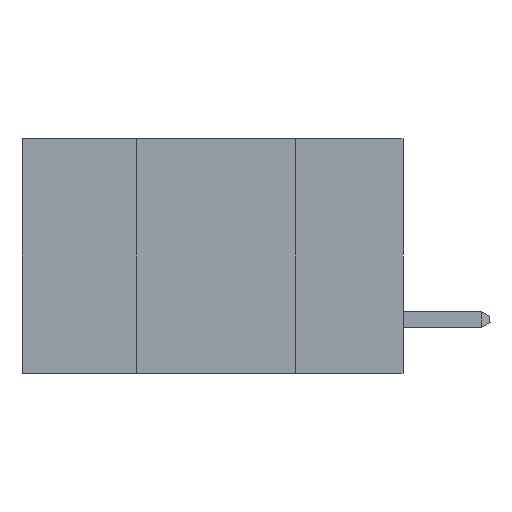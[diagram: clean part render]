
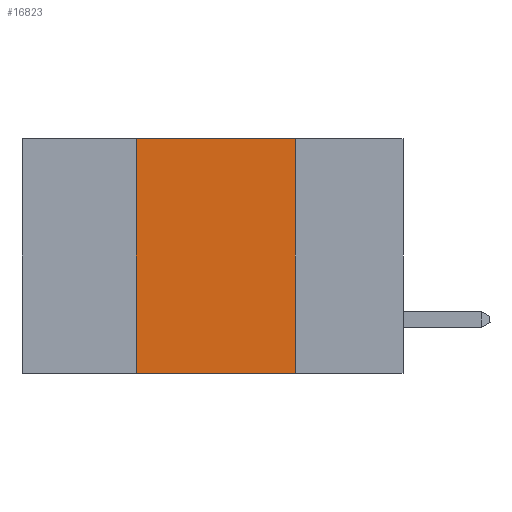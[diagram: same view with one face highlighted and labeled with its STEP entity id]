
A CAD part, left-side view. The second image highlights one B-rep face of the part: STEP entity #16823.
In plain terms, the highlighted planar face has unit normal (-1, 0, 0).
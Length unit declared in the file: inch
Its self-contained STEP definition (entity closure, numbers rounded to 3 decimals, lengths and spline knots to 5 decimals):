
#4189 = ORIENTED_EDGE ( 'NONE', *, *, #10110, .F. ) ;
#4251 = ORIENTED_EDGE ( 'NONE', *, *, #18059, .F. ) ;
#5193 = PLANE ( 'NONE',  #30608 ) ;
#5760 = DIRECTION ( 'NONE',  ( 0., -1., 0. ) ) ;
#8186 = VECTOR ( 'NONE', #33148, 39.37008 ) ;
#10110 = EDGE_CURVE ( 'NONE', #26115, #17063, #24623, .T. ) ;
#10211 = VECTOR ( 'NONE', #12003, 39.37008 ) ;
#12003 = DIRECTION ( 'NONE',  ( 0., 0., 1. ) ) ;
#16823 = ADVANCED_FACE ( 'NONE', ( #28544 ), #5193, .F. ) ;
#17063 = VERTEX_POINT ( 'NONE', #27699 ) ;
#18059 = EDGE_CURVE ( 'NONE', #17063, #22276, #43465, .T. ) ;
#20648 = DIRECTION ( 'NONE',  ( 0., 0., -1. ) ) ;
#21045 = VECTOR ( 'NONE', #36704, 39.37008 ) ;
#21968 = CARTESIAN_POINT ( 'NONE',  ( 0., 0.17, -0.37 ) ) ;
#22276 = VERTEX_POINT ( 'NONE', #21968 ) ;
#23095 = EDGE_LOOP ( 'NONE', ( #4251, #4189, #47231, #33267 ) ) ;
#23384 = CARTESIAN_POINT ( 'NONE',  ( 0., 0.42, 0. ) ) ;
#24623 = LINE ( 'NONE', #42435, #32812 ) ;
#26115 = VERTEX_POINT ( 'NONE', #38847 ) ;
#27699 = CARTESIAN_POINT ( 'NONE',  ( 0., 0.17, 0. ) ) ;
#28544 = FACE_OUTER_BOUND ( 'NONE', #23095, .T. ) ;
#29245 = CARTESIAN_POINT ( 'NONE',  ( 0., 0.17, 0. ) ) ;
#29698 = CARTESIAN_POINT ( 'NONE',  ( 0., 0.6, -0.37 ) ) ;
#30608 = AXIS2_PLACEMENT_3D ( 'NONE', #42679, #42826, #20648 ) ;
#32676 = LINE ( 'NONE', #29698, #21045 ) ;
#32812 = VECTOR ( 'NONE', #5760, 39.37008 ) ;
#33148 = DIRECTION ( 'NONE',  ( 0., 0., -1. ) ) ;
#33267 = ORIENTED_EDGE ( 'NONE', *, *, #37942, .T. ) ;
#36704 = DIRECTION ( 'NONE',  ( 0., -1., 0. ) ) ;
#36985 = EDGE_CURVE ( 'NONE', #47639, #26115, #43168, .T. ) ;
#37942 = EDGE_CURVE ( 'NONE', #47639, #22276, #32676, .T. ) ;
#38847 = CARTESIAN_POINT ( 'NONE',  ( 0., 0.42, 0. ) ) ;
#42435 = CARTESIAN_POINT ( 'NONE',  ( 0., 0.6, 0. ) ) ;
#42679 = CARTESIAN_POINT ( 'NONE',  ( 0., 0.6, 0. ) ) ;
#42826 = DIRECTION ( 'NONE',  ( 1., 0., 0. ) ) ;
#43168 = LINE ( 'NONE', #23384, #10211 ) ;
#43465 = LINE ( 'NONE', #29245, #8186 ) ;
#46519 = CARTESIAN_POINT ( 'NONE',  ( 0., 0.42, -0.37 ) ) ;
#47231 = ORIENTED_EDGE ( 'NONE', *, *, #36985, .F. ) ;
#47639 = VERTEX_POINT ( 'NONE', #46519 ) ;
